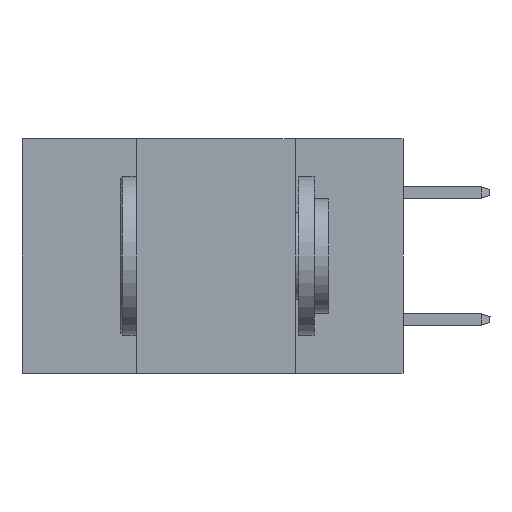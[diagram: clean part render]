
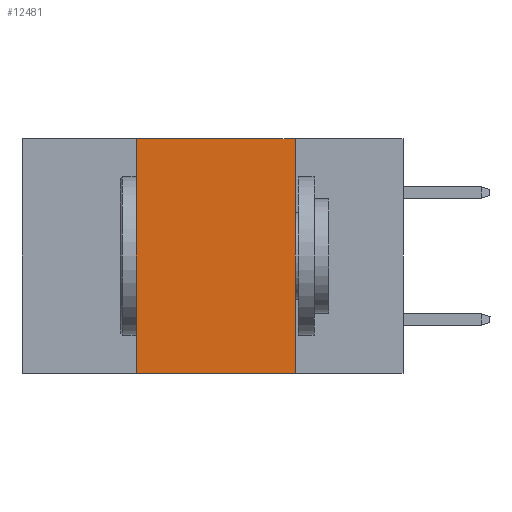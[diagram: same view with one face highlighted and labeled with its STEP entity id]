
A CAD part, left-side view. The second image highlights one B-rep face of the part: STEP entity #12481.
In plain terms, the highlighted planar face has unit normal (-1, 0, 0).
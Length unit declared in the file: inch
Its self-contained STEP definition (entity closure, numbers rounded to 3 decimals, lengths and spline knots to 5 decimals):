
#224 = DIRECTION ( 'NONE',  ( 0., 0., 1. ) ) ;
#320 = DIRECTION ( 'NONE',  ( 0., 0., -1. ) ) ;
#1684 = ORIENTED_EDGE ( 'NONE', *, *, #3457, .F. ) ;
#1797 = CARTESIAN_POINT ( 'NONE',  ( 0., 0.17, 0. ) ) ;
#2548 = ORIENTED_EDGE ( 'NONE', *, *, #8018, .F. ) ;
#2818 = VECTOR ( 'NONE', #224, 39.37008 ) ;
#2980 = VECTOR ( 'NONE', #18942, 39.37008 ) ;
#3043 = CARTESIAN_POINT ( 'NONE',  ( 0., 0.42, -0.37 ) ) ;
#3182 = LINE ( 'NONE', #15256, #2818 ) ;
#3457 = EDGE_CURVE ( 'NONE', #4004, #8588, #3182, .T. ) ;
#3741 = ORIENTED_EDGE ( 'NONE', *, *, #13799, .F. ) ;
#4004 = VERTEX_POINT ( 'NONE', #3043 ) ;
#4366 = CARTESIAN_POINT ( 'NONE',  ( 0., 0.6, 0. ) ) ;
#4755 = LINE ( 'NONE', #1797, #7409 ) ;
#5255 = CARTESIAN_POINT ( 'NONE',  ( 0., 0.6, -0.37 ) ) ;
#5786 = CARTESIAN_POINT ( 'NONE',  ( 0., 0.17, 0. ) ) ;
#7409 = VECTOR ( 'NONE', #320, 39.37008 ) ;
#8018 = EDGE_CURVE ( 'NONE', #13273, #12948, #4755, .T. ) ;
#8588 = VERTEX_POINT ( 'NONE', #9962 ) ;
#9471 = EDGE_CURVE ( 'NONE', #4004, #12948, #15773, .T. ) ;
#9729 = EDGE_LOOP ( 'NONE', ( #2548, #3741, #1684, #16977 ) ) ;
#9758 = VECTOR ( 'NONE', #10952, 39.37008 ) ;
#9852 = CARTESIAN_POINT ( 'NONE',  ( 0., 0.6, 0. ) ) ;
#9962 = CARTESIAN_POINT ( 'NONE',  ( 0., 0.42, 0. ) ) ;
#10952 = DIRECTION ( 'NONE',  ( 0., -1., 0. ) ) ;
#10994 = AXIS2_PLACEMENT_3D ( 'NONE', #4366, #12279, #18355 ) ;
#12279 = DIRECTION ( 'NONE',  ( 1., 0., 0. ) ) ;
#12481 = ADVANCED_FACE ( 'NONE', ( #16575 ), #17985, .F. ) ;
#12948 = VERTEX_POINT ( 'NONE', #16335 ) ;
#13273 = VERTEX_POINT ( 'NONE', #5786 ) ;
#13799 = EDGE_CURVE ( 'NONE', #8588, #13273, #14296, .T. ) ;
#14296 = LINE ( 'NONE', #9852, #9758 ) ;
#15256 = CARTESIAN_POINT ( 'NONE',  ( 0., 0.42, 0. ) ) ;
#15773 = LINE ( 'NONE', #5255, #2980 ) ;
#16335 = CARTESIAN_POINT ( 'NONE',  ( 0., 0.17, -0.37 ) ) ;
#16575 = FACE_OUTER_BOUND ( 'NONE', #9729, .T. ) ;
#16977 = ORIENTED_EDGE ( 'NONE', *, *, #9471, .T. ) ;
#17985 = PLANE ( 'NONE',  #10994 ) ;
#18355 = DIRECTION ( 'NONE',  ( 0., 0., -1. ) ) ;
#18942 = DIRECTION ( 'NONE',  ( 0., -1., 0. ) ) ;
